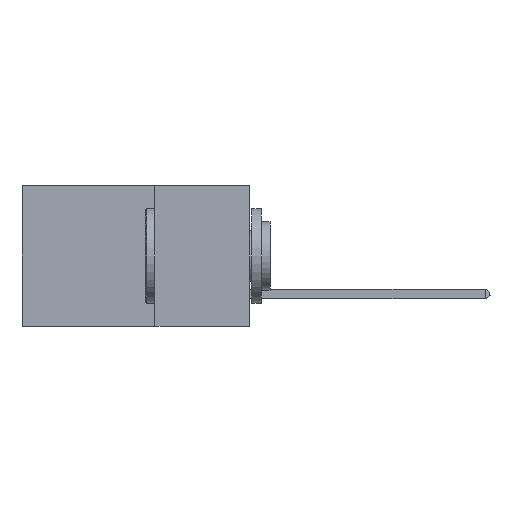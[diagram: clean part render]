
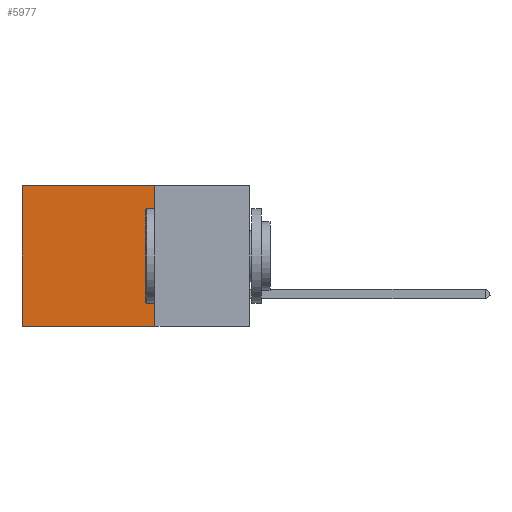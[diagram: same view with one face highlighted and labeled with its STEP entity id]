
A CAD part, left-side view. The second image highlights one B-rep face of the part: STEP entity #5977.
In plain terms, the highlighted planar face has unit normal (-1, 0, 0).
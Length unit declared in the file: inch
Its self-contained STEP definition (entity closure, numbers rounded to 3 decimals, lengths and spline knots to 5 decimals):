
#404 = CARTESIAN_POINT ( 'NONE',  ( 0.2875, 0.25, -0.37 ) ) ;
#655 = DIRECTION ( 'NONE',  ( 0., 0., -1. ) ) ;
#1389 = ORIENTED_EDGE ( 'NONE', *, *, #16007, .T. ) ;
#1756 = FACE_OUTER_BOUND ( 'NONE', #11088, .T. ) ;
#2075 = VECTOR ( 'NONE', #655, 39.37008 ) ;
#2464 = DIRECTION ( 'NONE',  ( 0., 0., -1. ) ) ;
#3405 = CARTESIAN_POINT ( 'NONE',  ( 0.2875, 0.25, -0.37 ) ) ;
#3940 = ORIENTED_EDGE ( 'NONE', *, *, #17414, .F. ) ;
#4408 = LINE ( 'NONE', #4709, #5057 ) ;
#4709 = CARTESIAN_POINT ( 'NONE',  ( 0.2875, 0.25, 0. ) ) ;
#5057 = VECTOR ( 'NONE', #16759, 39.37008 ) ;
#5105 = CARTESIAN_POINT ( 'NONE',  ( 0.2875, 0.25, 0. ) ) ;
#5113 = CARTESIAN_POINT ( 'NONE',  ( 0.2875, 0.6, -0.37 ) ) ;
#5209 = LINE ( 'NONE', #16451, #14487 ) ;
#5593 = EDGE_CURVE ( 'NONE', #14926, #15234, #5209, .T. ) ;
#5977 = ADVANCED_FACE ( 'NONE', ( #1756 ), #15607, .F. ) ;
#6259 = AXIS2_PLACEMENT_3D ( 'NONE', #5105, #13112, #2464 ) ;
#7075 = ORIENTED_EDGE ( 'NONE', *, *, #5593, .F. ) ;
#7415 = EDGE_CURVE ( 'NONE', #14926, #13956, #4408, .T. ) ;
#7933 = LINE ( 'NONE', #3405, #12522 ) ;
#10212 = VERTEX_POINT ( 'NONE', #5113 ) ;
#11088 = EDGE_LOOP ( 'NONE', ( #1389, #3940, #7075, #15528 ) ) ;
#11419 = CARTESIAN_POINT ( 'NONE',  ( 0.2875, 0.6, 0. ) ) ;
#12522 = VECTOR ( 'NONE', #16752, 39.37008 ) ;
#12799 = LINE ( 'NONE', #11419, #2075 ) ;
#13112 = DIRECTION ( 'NONE',  ( 1., 0., 0. ) ) ;
#13483 = DIRECTION ( 'NONE',  ( 0., 0., -1. ) ) ;
#13518 = CARTESIAN_POINT ( 'NONE',  ( 0.2875, 0.25, 0. ) ) ;
#13819 = CARTESIAN_POINT ( 'NONE',  ( 0.2875, 0.6, 0. ) ) ;
#13956 = VERTEX_POINT ( 'NONE', #13819 ) ;
#14487 = VECTOR ( 'NONE', #13483, 39.37008 ) ;
#14926 = VERTEX_POINT ( 'NONE', #13518 ) ;
#15234 = VERTEX_POINT ( 'NONE', #404 ) ;
#15528 = ORIENTED_EDGE ( 'NONE', *, *, #7415, .T. ) ;
#15607 = PLANE ( 'NONE',  #6259 ) ;
#16007 = EDGE_CURVE ( 'NONE', #13956, #10212, #12799, .T. ) ;
#16451 = CARTESIAN_POINT ( 'NONE',  ( 0.2875, 0.25, 0. ) ) ;
#16752 = DIRECTION ( 'NONE',  ( 0., 1., 0. ) ) ;
#16759 = DIRECTION ( 'NONE',  ( 0., 1., 0. ) ) ;
#17414 = EDGE_CURVE ( 'NONE', #15234, #10212, #7933, .T. ) ;
